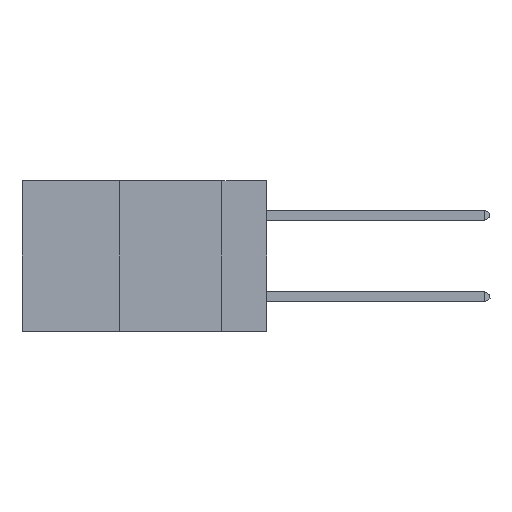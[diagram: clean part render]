
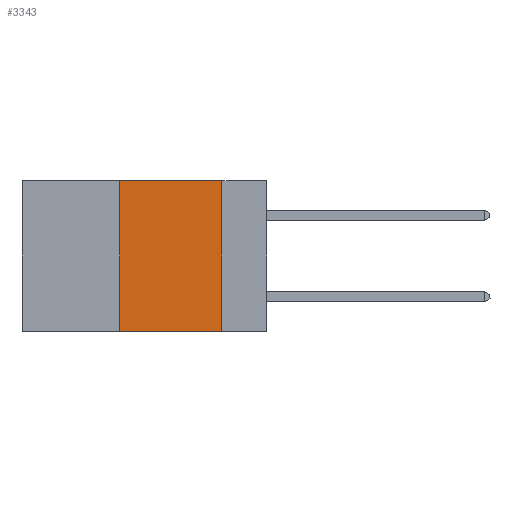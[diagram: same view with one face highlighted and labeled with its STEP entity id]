
A CAD part, left-side view. The second image highlights one B-rep face of the part: STEP entity #3343.
In plain terms, the highlighted planar face has unit normal (-1, 0, 0).
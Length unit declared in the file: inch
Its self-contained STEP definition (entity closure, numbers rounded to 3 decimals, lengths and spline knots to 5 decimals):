
#447 = EDGE_CURVE ( 'NONE', #7134, #2875, #5537, .T. ) ;
#1035 = DIRECTION ( 'NONE',  ( 0., 0., -1. ) ) ;
#1342 = LINE ( 'NONE', #11281, #3354 ) ;
#1783 = VECTOR ( 'NONE', #6865, 39.37008 ) ;
#2014 = VECTOR ( 'NONE', #7693, 39.37008 ) ;
#2811 = DIRECTION ( 'NONE',  ( 0., -1., 0. ) ) ;
#2875 = VERTEX_POINT ( 'NONE', #4499 ) ;
#3343 = ADVANCED_FACE ( 'NONE', ( #11063 ), #5564, .F. ) ;
#3354 = VECTOR ( 'NONE', #7853, 39.37008 ) ;
#4143 = LINE ( 'NONE', #13782, #1783 ) ;
#4499 = CARTESIAN_POINT ( 'NONE',  ( 0., 0.11, -0.37 ) ) ;
#5537 = LINE ( 'NONE', #10987, #13494 ) ;
#5564 = PLANE ( 'NONE',  #14089 ) ;
#6865 = DIRECTION ( 'NONE',  ( 0., -1., 0. ) ) ;
#7134 = VERTEX_POINT ( 'NONE', #7321 ) ;
#7321 = CARTESIAN_POINT ( 'NONE',  ( 0., 0.36, -0.37 ) ) ;
#7429 = LINE ( 'NONE', #11175, #2014 ) ;
#7693 = DIRECTION ( 'NONE',  ( 0., 0., -1. ) ) ;
#7853 = DIRECTION ( 'NONE',  ( 0., 0., 1. ) ) ;
#8081 = EDGE_CURVE ( 'NONE', #12983, #2875, #7429, .T. ) ;
#9065 = DIRECTION ( 'NONE',  ( 1., 0., 0. ) ) ;
#9136 = EDGE_CURVE ( 'NONE', #12004, #12983, #4143, .T. ) ;
#10206 = EDGE_LOOP ( 'NONE', ( #14117, #13554, #11866, #13560 ) ) ;
#10377 = CARTESIAN_POINT ( 'NONE',  ( 0., 0.11, 0. ) ) ;
#10987 = CARTESIAN_POINT ( 'NONE',  ( 0., 0.6, -0.37 ) ) ;
#11063 = FACE_OUTER_BOUND ( 'NONE', #10206, .T. ) ;
#11175 = CARTESIAN_POINT ( 'NONE',  ( 0., 0.11, 0. ) ) ;
#11281 = CARTESIAN_POINT ( 'NONE',  ( 0., 0.36, 0. ) ) ;
#11866 = ORIENTED_EDGE ( 'NONE', *, *, #14371, .F. ) ;
#12004 = VERTEX_POINT ( 'NONE', #12245 ) ;
#12245 = CARTESIAN_POINT ( 'NONE',  ( 0., 0.36, 0. ) ) ;
#12983 = VERTEX_POINT ( 'NONE', #10377 ) ;
#13494 = VECTOR ( 'NONE', #2811, 39.37008 ) ;
#13554 = ORIENTED_EDGE ( 'NONE', *, *, #9136, .F. ) ;
#13560 = ORIENTED_EDGE ( 'NONE', *, *, #447, .T. ) ;
#13782 = CARTESIAN_POINT ( 'NONE',  ( 0., 0.6, 0. ) ) ;
#14089 = AXIS2_PLACEMENT_3D ( 'NONE', #14810, #9065, #1035 ) ;
#14117 = ORIENTED_EDGE ( 'NONE', *, *, #8081, .F. ) ;
#14371 = EDGE_CURVE ( 'NONE', #7134, #12004, #1342, .T. ) ;
#14810 = CARTESIAN_POINT ( 'NONE',  ( 0., 0.6, 0. ) ) ;
